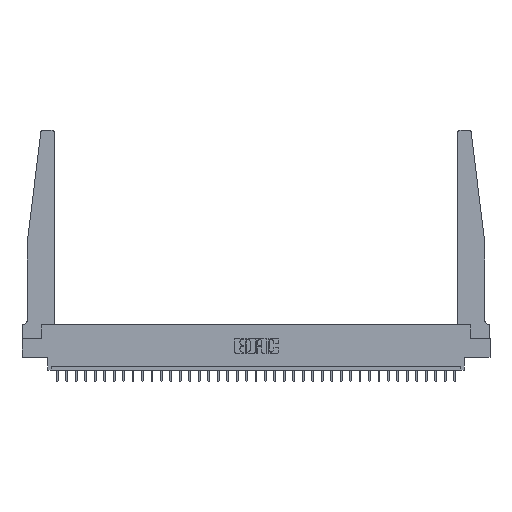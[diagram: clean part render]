
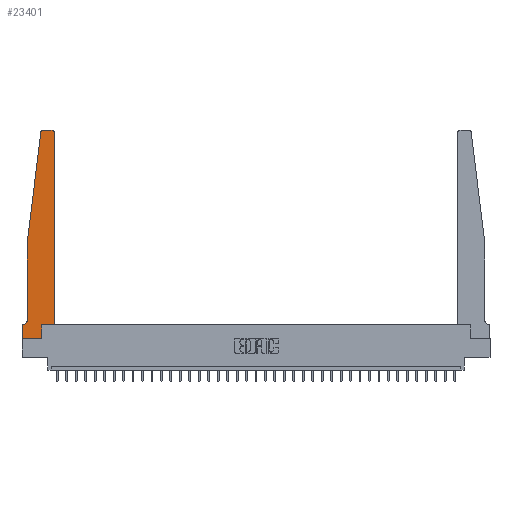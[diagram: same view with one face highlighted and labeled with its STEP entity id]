
A CAD part, top view. The second image highlights one B-rep face of the part: STEP entity #23401.
In plain terms, the highlighted planar face has unit normal (0, 0, 1).
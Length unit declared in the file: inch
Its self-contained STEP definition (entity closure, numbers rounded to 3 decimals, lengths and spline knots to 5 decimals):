
#68 = FACE_OUTER_BOUND ( 'NONE', #9089, .T. ) ;
#240 = VECTOR ( 'NONE', #2293, 39.37008 ) ;
#247 = CARTESIAN_POINT ( 'NONE',  ( 0.065, 0.1875, 0.37 ) ) ;
#352 = VECTOR ( 'NONE', #19732, 39.37008 ) ;
#482 = AXIS2_PLACEMENT_3D ( 'NONE', #11968, #17139, #26679 ) ;
#549 = CARTESIAN_POINT ( 'NONE',  ( 0., 0.1875, 0.37 ) ) ;
#680 = DIRECTION ( 'NONE',  ( 0., 0., 1. ) ) ;
#1108 = CARTESIAN_POINT ( 'NONE',  ( 0., 0., 0.37 ) ) ;
#1174 = ORIENTED_EDGE ( 'NONE', *, *, #18672, .T. ) ;
#1241 = EDGE_CURVE ( 'NONE', #18714, #30985, #12320, .T. ) ;
#1464 = VECTOR ( 'NONE', #10255, 39.37008 ) ;
#2135 = DIRECTION ( 'NONE',  ( 0., 1., 0. ) ) ;
#2200 = LINE ( 'NONE', #12056, #17448 ) ;
#2293 = DIRECTION ( 'NONE',  ( 0., -1., 0. ) ) ;
#2324 = ORIENTED_EDGE ( 'NONE', *, *, #29446, .T. ) ;
#2496 = ORIENTED_EDGE ( 'NONE', *, *, #28161, .T. ) ;
#3115 = CARTESIAN_POINT ( 'NONE',  ( 0.425, 2.72, 0.37 ) ) ;
#3280 = CARTESIAN_POINT ( 'NONE',  ( 0., 0.1875, 0.37 ) ) ;
#3337 = CARTESIAN_POINT ( 'NONE',  ( 0.395, 2.72, 0.37 ) ) ;
#4127 = LINE ( 'NONE', #1108, #14909 ) ;
#4568 = DIRECTION ( 'NONE',  ( -1., 0., 0. ) ) ;
#4572 = CARTESIAN_POINT ( 'NONE',  ( 0.27653, 2.75, 0.37 ) ) ;
#4619 = LINE ( 'NONE', #21278, #12178 ) ;
#5039 = DIRECTION ( 'NONE',  ( 0., 0., 1. ) ) ;
#5522 = LINE ( 'NONE', #5682, #6845 ) ;
#5553 = ORIENTED_EDGE ( 'NONE', *, *, #17727, .T. ) ;
#5596 = VERTEX_POINT ( 'NONE', #15252 ) ;
#5682 = CARTESIAN_POINT ( 'NONE',  ( 0.065, 1.25, 0.37 ) ) ;
#6211 = VERTEX_POINT ( 'NONE', #22651 ) ;
#6845 = VECTOR ( 'NONE', #25259, 39.37008 ) ;
#8103 = ORIENTED_EDGE ( 'NONE', *, *, #13505, .T. ) ;
#9089 = EDGE_LOOP ( 'NONE', ( #10258, #28098, #2324, #1174, #5553, #21280, #14088, #28493, #31368, #2496, #8103, #19962 ) ) ;
#9892 = PLANE ( 'NONE',  #13015 ) ;
#10255 = DIRECTION ( 'NONE',  ( 0., -1., 0. ) ) ;
#10258 = ORIENTED_EDGE ( 'NONE', *, *, #18461, .T. ) ;
#10758 = VERTEX_POINT ( 'NONE', #25854 ) ;
#11968 = CARTESIAN_POINT ( 'NONE',  ( 0.015, 0.2375, 0.37 ) ) ;
#12056 = CARTESIAN_POINT ( 'NONE',  ( 0.25, 2.75, 0.37 ) ) ;
#12178 = VECTOR ( 'NONE', #16434, 39.37008 ) ;
#12320 = LINE ( 'NONE', #22161, #352 ) ;
#12377 = CARTESIAN_POINT ( 'NONE',  ( 0.2605, 0., 0.37 ) ) ;
#12494 = LINE ( 'NONE', #247, #13151 ) ;
#12776 = DIRECTION ( 'NONE',  ( 1., 0., 0. ) ) ;
#13015 = AXIS2_PLACEMENT_3D ( 'NONE', #549, #5039, #24766 ) ;
#13151 = VECTOR ( 'NONE', #4568, 39.37008 ) ;
#13505 = EDGE_CURVE ( 'NONE', #5596, #30776, #24272, .T. ) ;
#13995 = CARTESIAN_POINT ( 'NONE',  ( 0.065, 1.25, 0.37 ) ) ;
#14088 = ORIENTED_EDGE ( 'NONE', *, *, #29694, .T. ) ;
#14557 = LINE ( 'NONE', #14721, #240 ) ;
#14721 = CARTESIAN_POINT ( 'NONE',  ( 0., 0., 0.37 ) ) ;
#14909 = VECTOR ( 'NONE', #28385, 39.37008 ) ;
#15252 = CARTESIAN_POINT ( 'NONE',  ( 0.425, 0.18, 0.37 ) ) ;
#15994 = AXIS2_PLACEMENT_3D ( 'NONE', #27324, #680, #12776 ) ;
#16434 = DIRECTION ( 'NONE',  ( 1., 0., 0. ) ) ;
#17139 = DIRECTION ( 'NONE',  ( 0., 0., -1. ) ) ;
#17148 = CARTESIAN_POINT ( 'NONE',  ( 0.2605, 0.18, 0.37 ) ) ;
#17312 = CARTESIAN_POINT ( 'NONE',  ( 0.425, 0.18, 0.37 ) ) ;
#17448 = VECTOR ( 'NONE', #21738, 39.37008 ) ;
#17727 = EDGE_CURVE ( 'NONE', #10758, #24354, #22104, .T. ) ;
#18001 = CARTESIAN_POINT ( 'NONE',  ( 0.065, 1.25, 0.37 ) ) ;
#18376 = EDGE_CURVE ( 'NONE', #18575, #18714, #4127, .T. ) ;
#18461 = EDGE_CURVE ( 'NONE', #27985, #27069, #2200, .T. ) ;
#18575 = VERTEX_POINT ( 'NONE', #29008 ) ;
#18672 = EDGE_CURVE ( 'NONE', #19723, #10758, #25296, .T. ) ;
#18714 = VERTEX_POINT ( 'NONE', #12377 ) ;
#19723 = VERTEX_POINT ( 'NONE', #13995 ) ;
#19732 = DIRECTION ( 'NONE',  ( 0., 1., 0. ) ) ;
#19962 = ORIENTED_EDGE ( 'NONE', *, *, #21347, .T. ) ;
#20828 = EDGE_CURVE ( 'NONE', #27069, #6211, #24239, .T. ) ;
#21154 = CIRCLE ( 'NONE', #29943, 0.03 ) ;
#21278 = CARTESIAN_POINT ( 'NONE',  ( 0.425, 0.18, 0.37 ) ) ;
#21280 = ORIENTED_EDGE ( 'NONE', *, *, #30634, .T. ) ;
#21347 = EDGE_CURVE ( 'NONE', #30776, #27985, #21154, .T. ) ;
#21738 = DIRECTION ( 'NONE',  ( -1., 0., 0. ) ) ;
#22104 = CIRCLE ( 'NONE', #482, 0.05 ) ;
#22161 = CARTESIAN_POINT ( 'NONE',  ( 0.2605, 0.18, 0.37 ) ) ;
#22651 = CARTESIAN_POINT ( 'NONE',  ( 0.24675, 2.72367, 0.37 ) ) ;
#23224 = DIRECTION ( 'NONE',  ( 0., 0., 1. ) ) ;
#23401 = ADVANCED_FACE ( 'NONE', ( #68 ), #9892, .T. ) ;
#24239 = CIRCLE ( 'NONE', #15994, 0.03 ) ;
#24272 = LINE ( 'NONE', #17312, #25769 ) ;
#24354 = VERTEX_POINT ( 'NONE', #25758 ) ;
#24766 = DIRECTION ( 'NONE',  ( 1., 0., 0. ) ) ;
#25259 = DIRECTION ( 'NONE',  ( -0.122, -0.992, 0. ) ) ;
#25296 = LINE ( 'NONE', #18001, #1464 ) ;
#25758 = CARTESIAN_POINT ( 'NONE',  ( 0.015, 0.1875, 0.37 ) ) ;
#25769 = VECTOR ( 'NONE', #2135, 39.37008 ) ;
#25854 = CARTESIAN_POINT ( 'NONE',  ( 0.065, 0.2375, 0.37 ) ) ;
#26679 = DIRECTION ( 'NONE',  ( -1., 0., 0. ) ) ;
#27069 = VERTEX_POINT ( 'NONE', #4572 ) ;
#27076 = VERTEX_POINT ( 'NONE', #3280 ) ;
#27324 = CARTESIAN_POINT ( 'NONE',  ( 0.27653, 2.72, 0.37 ) ) ;
#27985 = VERTEX_POINT ( 'NONE', #30804 ) ;
#28098 = ORIENTED_EDGE ( 'NONE', *, *, #20828, .T. ) ;
#28161 = EDGE_CURVE ( 'NONE', #30985, #5596, #4619, .T. ) ;
#28385 = DIRECTION ( 'NONE',  ( 1., 0., 0. ) ) ;
#28493 = ORIENTED_EDGE ( 'NONE', *, *, #18376, .T. ) ;
#29008 = CARTESIAN_POINT ( 'NONE',  ( 0., 0., 0.37 ) ) ;
#29446 = EDGE_CURVE ( 'NONE', #6211, #19723, #5522, .T. ) ;
#29694 = EDGE_CURVE ( 'NONE', #27076, #18575, #14557, .T. ) ;
#29943 = AXIS2_PLACEMENT_3D ( 'NONE', #3337, #23224, #30956 ) ;
#30634 = EDGE_CURVE ( 'NONE', #24354, #27076, #12494, .T. ) ;
#30776 = VERTEX_POINT ( 'NONE', #3115 ) ;
#30804 = CARTESIAN_POINT ( 'NONE',  ( 0.395, 2.75, 0.37 ) ) ;
#30956 = DIRECTION ( 'NONE',  ( 1., 0., 0. ) ) ;
#30985 = VERTEX_POINT ( 'NONE', #17148 ) ;
#31368 = ORIENTED_EDGE ( 'NONE', *, *, #1241, .T. ) ;
